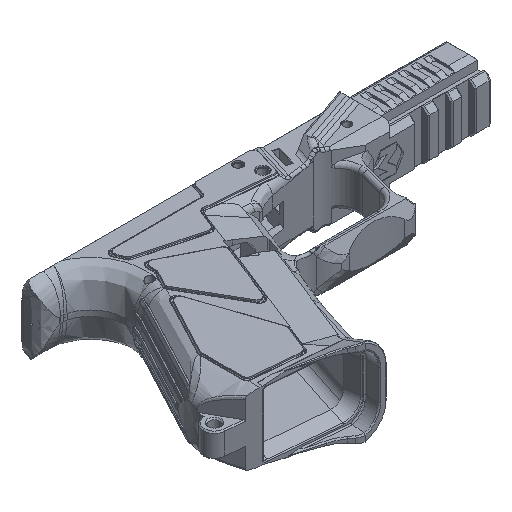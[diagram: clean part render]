
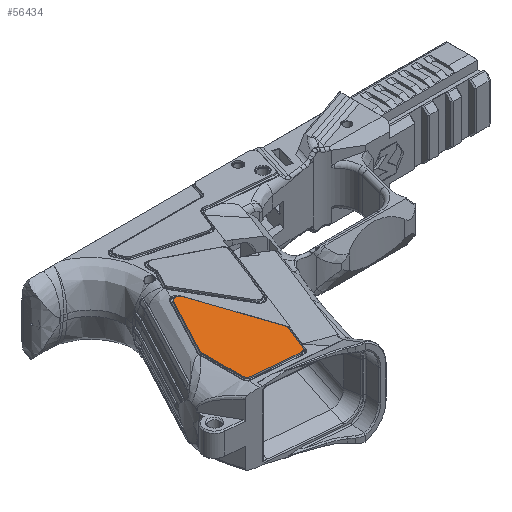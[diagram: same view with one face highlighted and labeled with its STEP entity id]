
A CAD part, isometric view. The second image highlights one B-rep face of the part: STEP entity #56434.
In plain terms, the highlighted planar face has unit normal (0, 0, 1).
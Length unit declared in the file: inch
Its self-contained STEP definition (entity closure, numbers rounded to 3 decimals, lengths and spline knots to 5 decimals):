
#607 = AXIS2_PLACEMENT_3D ( 'NONE', #62065, #4093, #9202 ) ;
#2817 = VERTEX_POINT ( 'NONE', #16050 ) ;
#2985 = DIRECTION ( 'NONE',  ( 0., 0., 1. ) ) ;
#3176 = VERTEX_POINT ( 'NONE', #80071 ) ;
#3860 = DIRECTION ( 'NONE',  ( 0., 0., 1. ) ) ;
#4093 = DIRECTION ( 'NONE',  ( 0., 0., 1. ) ) ;
#4641 = VERTEX_POINT ( 'NONE', #77855 ) ;
#4827 = CARTESIAN_POINT ( 'NONE',  ( 0.11818, -2.59557, 0.58693 ) ) ;
#9005 = EDGE_CURVE ( 'NONE', #42103, #4641, #77447, .T. ) ;
#9202 = DIRECTION ( 'NONE',  ( 1., 0., 0. ) ) ;
#9869 = DIRECTION ( 'NONE',  ( 1., 0., 0. ) ) ;
#12222 = CARTESIAN_POINT ( 'NONE',  ( 0.76992, -1.65722, 0.58693 ) ) ;
#13265 = DIRECTION ( 'NONE',  ( 0.367, 0.93, 0. ) ) ;
#13537 = VERTEX_POINT ( 'NONE', #27431 ) ;
#14153 = CARTESIAN_POINT ( 'NONE',  ( 0.69412, -1.68279, 0.58693 ) ) ;
#14530 = CARTESIAN_POINT ( 'NONE',  ( 1.1221, -2.95116, 0.58693 ) ) ;
#15018 = CARTESIAN_POINT ( 'NONE',  ( 1.1979, -2.92558, 0.58693 ) ) ;
#16050 = CARTESIAN_POINT ( 'NONE',  ( 1.19653, -2.98048, 0.58693 ) ) ;
#17060 = ORIENTED_EDGE ( 'NONE', *, *, #32524, .T. ) ;
#18058 = CARTESIAN_POINT ( 'NONE',  ( 0.19818, -2.61552, 0.58693 ) ) ;
#18094 = EDGE_CURVE ( 'NONE', #73762, #43604, #24752, .T. ) ;
#19167 = CARTESIAN_POINT ( 'NONE',  ( 0.95138, -3.44617, 0.58693 ) ) ;
#19670 = CARTESIAN_POINT ( 'NONE',  ( 0.82976, -1.83457, 0.58693 ) ) ;
#19824 = ORIENTED_EDGE ( 'NONE', *, *, #21131, .T. ) ;
#20960 = CARTESIAN_POINT ( 'NONE',  ( 0.11818, -3.3718, 0.58693 ) ) ;
#21131 = EDGE_CURVE ( 'NONE', #13537, #2817, #60220, .T. ) ;
#22279 = CIRCLE ( 'NONE', #24971, 0.08 ) ;
#22881 = DIRECTION ( 'NONE',  ( 1., 0., 0. ) ) ;
#23564 = CIRCLE ( 'NONE', #51970, 0.08 ) ;
#24029 = ORIENTED_EDGE ( 'NONE', *, *, #72016, .T. ) ;
#24205 = AXIS2_PLACEMENT_3D ( 'NONE', #55056, #3860, #22881 ) ;
#24752 = CIRCLE ( 'NONE', #72061, 0.08 ) ;
#24904 = LINE ( 'NONE', #20960, #62194 ) ;
#24971 = AXIS2_PLACEMENT_3D ( 'NONE', #14530, #33954, #9869 ) ;
#25397 = CARTESIAN_POINT ( 'NONE',  ( 0.12754, -2.57796, 0.58693 ) ) ;
#25683 = PLANE ( 'NONE',  #51179 ) ;
#26089 = ORIENTED_EDGE ( 'NONE', *, *, #9005, .T. ) ;
#27431 = CARTESIAN_POINT ( 'NONE',  ( 1.03293, -3.39581, 0.58693 ) ) ;
#27433 = EDGE_CURVE ( 'NONE', #62667, #13537, #66884, .T. ) ;
#29681 = CARTESIAN_POINT ( 'NONE',  ( 1.2021, -2.95116, 0.58693 ) ) ;
#29865 = DIRECTION ( 'NONE',  ( -0.469, -0.883, 0. ) ) ;
#31019 = LINE ( 'NONE', #4827, #68826 ) ;
#32524 = EDGE_CURVE ( 'NONE', #2817, #80362, #22279, .T. ) ;
#33004 = CARTESIAN_POINT ( 'NONE',  ( 0.11818, -3.29862, 0.58693 ) ) ;
#33158 = DIRECTION ( 'NONE',  ( 0., 0., 1. ) ) ;
#33954 = DIRECTION ( 'NONE',  ( 0., 0., 1. ) ) ;
#34111 = FACE_OUTER_BOUND ( 'NONE', #67360, .T. ) ;
#34679 = CARTESIAN_POINT ( 'NONE',  ( 0.19818, -3.29862, 0.58693 ) ) ;
#35807 = VECTOR ( 'NONE', #29865, 39.37008 ) ;
#36626 = LINE ( 'NONE', #68391, #35807 ) ;
#37760 = DIRECTION ( 'NONE',  ( 0., -1., 0. ) ) ;
#38193 = AXIS2_PLACEMENT_3D ( 'NONE', #18058, #45070, #77263 ) ;
#39074 = DIRECTION ( 'NONE',  ( 1., 0., 0. ) ) ;
#40127 = VECTOR ( 'NONE', #13265, 39.37008 ) ;
#41302 = CARTESIAN_POINT ( 'NONE',  ( 5.22366, -0.35196, 0.58693 ) ) ;
#42103 = VERTEX_POINT ( 'NONE', #25397 ) ;
#43604 = VERTEX_POINT ( 'NONE', #52855 ) ;
#44611 = EDGE_CURVE ( 'NONE', #80362, #57540, #83660, .T. ) ;
#45070 = DIRECTION ( 'NONE',  ( 0., 0., 1. ) ) ;
#47817 = DIRECTION ( 'NONE',  ( 1., 0., 0. ) ) ;
#51143 = DIRECTION ( 'NONE',  ( 0.996, -0.089, 0. ) ) ;
#51179 = AXIS2_PLACEMENT_3D ( 'NONE', #41302, #61215, #54032 ) ;
#51970 = AXIS2_PLACEMENT_3D ( 'NONE', #34679, #2985, #47817 ) ;
#52235 = ORIENTED_EDGE ( 'NONE', *, *, #27433, .T. ) ;
#52339 = ORIENTED_EDGE ( 'NONE', *, *, #68208, .T. ) ;
#52855 = CARTESIAN_POINT ( 'NONE',  ( 0.62348, -1.64524, 0.58693 ) ) ;
#53864 = CARTESIAN_POINT ( 'NONE',  ( 1.01099, -3.45149, 0.58693 ) ) ;
#54032 = DIRECTION ( 'NONE',  ( 1., 0., 0. ) ) ;
#55056 = CARTESIAN_POINT ( 'NONE',  ( 1.1221, -2.95116, 0.58693 ) ) ;
#55991 = ORIENTED_EDGE ( 'NONE', *, *, #80927, .T. ) ;
#56434 = ADVANCED_FACE ( 'NONE', ( #34111 ), #25683, .T. ) ;
#57540 = VERTEX_POINT ( 'NONE', #15018 ) ;
#58611 = LINE ( 'NONE', #19670, #61467 ) ;
#60220 = LINE ( 'NONE', #53864, #40127 ) ;
#60301 = ORIENTED_EDGE ( 'NONE', *, *, #18094, .T. ) ;
#61215 = DIRECTION ( 'NONE',  ( 0., 0., 1. ) ) ;
#61467 = VECTOR ( 'NONE', #78062, 39.37008 ) ;
#62065 = CARTESIAN_POINT ( 'NONE',  ( 0.9585, -3.36649, 0.58693 ) ) ;
#62194 = VECTOR ( 'NONE', #51143, 39.37008 ) ;
#62667 = VERTEX_POINT ( 'NONE', #19167 ) ;
#66884 = CIRCLE ( 'NONE', #607, 0.08 ) ;
#67360 = EDGE_LOOP ( 'NONE', ( #19824, #17060, #80909, #83638, #60301, #24029, #26089, #73590, #52339, #55991, #52235 ) ) ;
#68208 = EDGE_CURVE ( 'NONE', #80444, #3176, #23564, .T. ) ;
#68391 = CARTESIAN_POINT ( 'NONE',  ( 0.92714, -1.07414, 0.58693 ) ) ;
#68826 = VECTOR ( 'NONE', #37760, 39.37008 ) ;
#71272 = EDGE_CURVE ( 'NONE', #57540, #73762, #58611, .T. ) ;
#72016 = EDGE_CURVE ( 'NONE', #43604, #42103, #36626, .T. ) ;
#72061 = AXIS2_PLACEMENT_3D ( 'NONE', #14153, #33158, #39074 ) ;
#73590 = ORIENTED_EDGE ( 'NONE', *, *, #78802, .T. ) ;
#73762 = VERTEX_POINT ( 'NONE', #12222 ) ;
#77263 = DIRECTION ( 'NONE',  ( 1., 0., 0. ) ) ;
#77447 = CIRCLE ( 'NONE', #38193, 0.08 ) ;
#77855 = CARTESIAN_POINT ( 'NONE',  ( 0.11818, -2.61552, 0.58693 ) ) ;
#78062 = DIRECTION ( 'NONE',  ( -0.32, 0.948, 0. ) ) ;
#78802 = EDGE_CURVE ( 'NONE', #4641, #80444, #31019, .T. ) ;
#80071 = CARTESIAN_POINT ( 'NONE',  ( 0.19107, -3.3783, 0.58693 ) ) ;
#80362 = VERTEX_POINT ( 'NONE', #29681 ) ;
#80444 = VERTEX_POINT ( 'NONE', #33004 ) ;
#80909 = ORIENTED_EDGE ( 'NONE', *, *, #44611, .T. ) ;
#80927 = EDGE_CURVE ( 'NONE', #3176, #62667, #24904, .T. ) ;
#83638 = ORIENTED_EDGE ( 'NONE', *, *, #71272, .T. ) ;
#83660 = CIRCLE ( 'NONE', #24205, 0.08 ) ;
